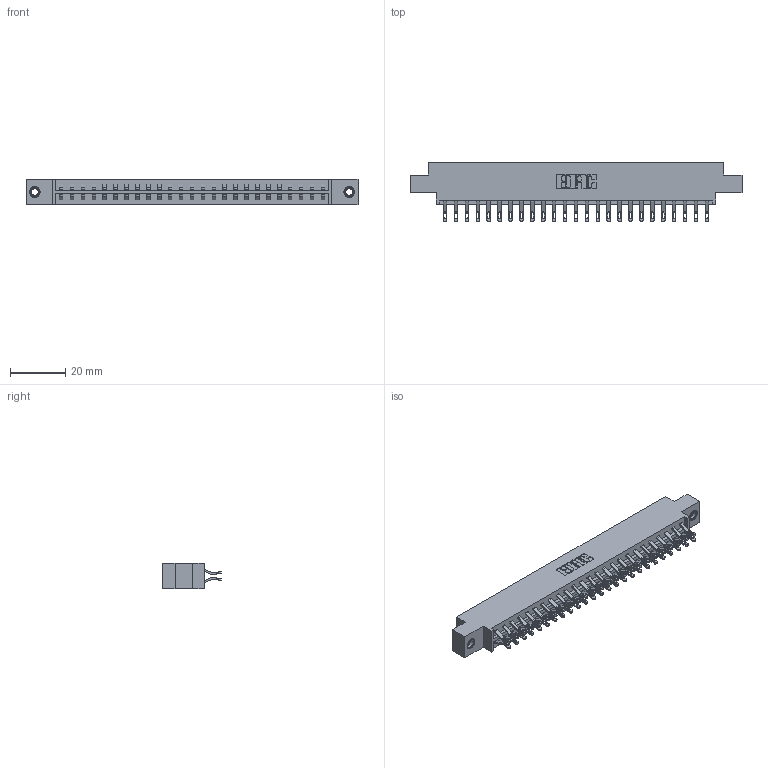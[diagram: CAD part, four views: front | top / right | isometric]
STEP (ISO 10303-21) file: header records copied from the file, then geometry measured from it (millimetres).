
FILE_DESCRIPTION (( 'STEP AP203' ), '1' );
FILE_NAME ('833-050-555-807.STEP', '2020-06-04T18:01:44', ( '' ), ( '' ), 'SwSTEP 2.0', 'SolidWorks 2020', '' );
FILE_SCHEMA (( 'CONFIG_CONTROL_DESIGN' ));
Length unit declared in the file: inch
Products named in the file (4): 833 Part_Offset - .156 Dia - TI; 833-050-555-807; 345-250-001_345-250-005-103; 345-292-001_555 Tail
Assembly tree (53 placements, depth 2):
  833-050-555-807
    833 Part_Offset - .156 Dia - TI
    345-292-001_555 Tail  x50
    345-250-001_345-250-005-103  x2
Bounding box: 120.6 x 21.47 x 9.4 mm (x, y, z)
Volume: 12057.2 mm3; surface area: 14869.3 mm2
Topology: 53 solids, 53 shells, 3078 faces, 9609 edges, 6398 vertices
Faces by surface type: plane 1806, cylinder 1256, cone 12, torus 4
Entity records: 19926 total; most frequent: CARTESIAN_POINT 3343, ORIENTED_EDGE 3242, DIRECTION 2887, EDGE_CURVE 1621, LINE 1453, VECTOR 1453, VERTEX_POINT 1076, AXIS2_PLACEMENT_3D 717
